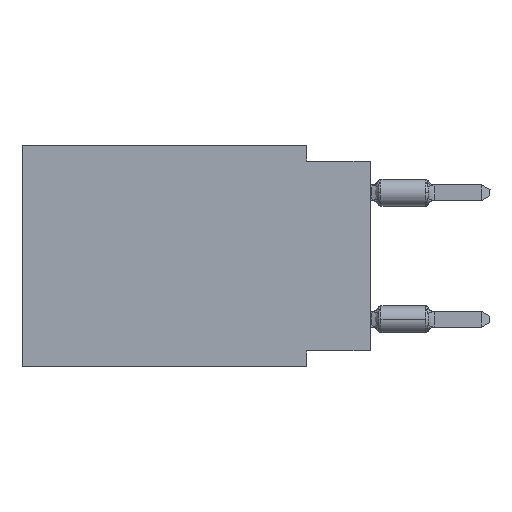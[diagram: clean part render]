
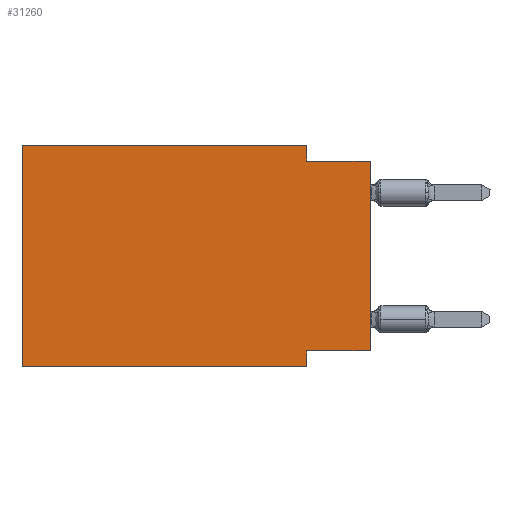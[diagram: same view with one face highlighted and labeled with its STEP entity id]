
A CAD part, left-side view. The second image highlights one B-rep face of the part: STEP entity #31260.
In plain terms, the highlighted planar face has unit normal (-1, 0, 0).
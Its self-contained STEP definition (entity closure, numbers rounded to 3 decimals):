
#143 = DIRECTION ( 'NONE',  ( 0., -1., 0. ) ) ;
#1596 = LINE ( 'NONE', #15163, #25583 ) ;
#1943 = EDGE_CURVE ( 'NONE', #33168, #24580, #10604, .T. ) ;
#2580 = FACE_OUTER_BOUND ( 'NONE', #4321, .T. ) ;
#3035 = VECTOR ( 'NONE', #9583, 1000. ) ;
#3718 = EDGE_CURVE ( 'NONE', #33021, #20253, #37984, .T. ) ;
#4321 = EDGE_LOOP ( 'NONE', ( #15997, #19466, #8358, #24351, #36821, #16368, #6652, #5869 ) ) ;
#4835 = DIRECTION ( 'NONE',  ( 0., 0., -1. ) ) ;
#5869 = ORIENTED_EDGE ( 'NONE', *, *, #16274, .F. ) ;
#6652 = ORIENTED_EDGE ( 'NONE', *, *, #42197, .F. ) ;
#6726 = CARTESIAN_POINT ( 'NONE',  ( 0., 2.54, -8.255 ) ) ;
#7044 = VECTOR ( 'NONE', #23242, 1000. ) ;
#8358 = ORIENTED_EDGE ( 'NONE', *, *, #13438, .F. ) ;
#8679 = VECTOR ( 'NONE', #29029, 1000. ) ;
#8822 = PLANE ( 'NONE',  #34450 ) ;
#9538 = CARTESIAN_POINT ( 'NONE',  ( 0., 2.54, -0.635 ) ) ;
#9583 = DIRECTION ( 'NONE',  ( 0., -1., 0. ) ) ;
#10604 = LINE ( 'NONE', #37695, #11522 ) ;
#11522 = VECTOR ( 'NONE', #143, 1000. ) ;
#11567 = LINE ( 'NONE', #34256, #15675 ) ;
#13027 = DIRECTION ( 'NONE',  ( 1., 0., 0. ) ) ;
#13438 = EDGE_CURVE ( 'NONE', #24580, #42688, #38391, .T. ) ;
#13461 = LINE ( 'NONE', #16352, #7044 ) ;
#14461 = DIRECTION ( 'NONE',  ( 0., 0., -1. ) ) ;
#15055 = CARTESIAN_POINT ( 'NONE',  ( 0., 2.54, 0. ) ) ;
#15163 = CARTESIAN_POINT ( 'NONE',  ( 0., 13.97, 0. ) ) ;
#15467 = CARTESIAN_POINT ( 'NONE',  ( 0., 0., 0. ) ) ;
#15601 = DIRECTION ( 'NONE',  ( 0., 1., 0. ) ) ;
#15675 = VECTOR ( 'NONE', #14461, 1000. ) ;
#15825 = CARTESIAN_POINT ( 'NONE',  ( 0., 0., -8.255 ) ) ;
#15997 = ORIENTED_EDGE ( 'NONE', *, *, #3718, .T. ) ;
#16274 = EDGE_CURVE ( 'NONE', #33021, #35080, #36049, .T. ) ;
#16352 = CARTESIAN_POINT ( 'NONE',  ( 0., 0., -0.635 ) ) ;
#16368 = ORIENTED_EDGE ( 'NONE', *, *, #20958, .T. ) ;
#18544 = CARTESIAN_POINT ( 'NONE',  ( 0., 13.97, -8.89 ) ) ;
#19466 = ORIENTED_EDGE ( 'NONE', *, *, #28152, .F. ) ;
#20253 = VERTEX_POINT ( 'NONE', #22331 ) ;
#20958 = EDGE_CURVE ( 'NONE', #43331, #32548, #36255, .T. ) ;
#22331 = CARTESIAN_POINT ( 'NONE',  ( 0., 0., -0.635 ) ) ;
#23242 = DIRECTION ( 'NONE',  ( 0., -1., 0. ) ) ;
#24351 = ORIENTED_EDGE ( 'NONE', *, *, #1943, .F. ) ;
#24580 = VERTEX_POINT ( 'NONE', #38920 ) ;
#24868 = VECTOR ( 'NONE', #4835, 1000. ) ;
#25583 = VECTOR ( 'NONE', #38922, 1000. ) ;
#26576 = DIRECTION ( 'NONE',  ( 0., 0., -1. ) ) ;
#26583 = CARTESIAN_POINT ( 'NONE',  ( 0., 2.54, -8.89 ) ) ;
#28152 = EDGE_CURVE ( 'NONE', #42688, #20253, #13461, .T. ) ;
#29029 = DIRECTION ( 'NONE',  ( 0., 0., 1. ) ) ;
#29907 = CARTESIAN_POINT ( 'NONE',  ( 0., 13.97, 0. ) ) ;
#31260 = ADVANCED_FACE ( 'NONE', ( #2580 ), #8822, .F. ) ;
#32548 = VERTEX_POINT ( 'NONE', #26583 ) ;
#33021 = VERTEX_POINT ( 'NONE', #40290 ) ;
#33168 = VERTEX_POINT ( 'NONE', #42041 ) ;
#34256 = CARTESIAN_POINT ( 'NONE',  ( 0., 2.54, -8.89 ) ) ;
#34450 = AXIS2_PLACEMENT_3D ( 'NONE', #29907, #13027, #26576 ) ;
#35080 = VERTEX_POINT ( 'NONE', #6726 ) ;
#36049 = LINE ( 'NONE', #15825, #37717 ) ;
#36255 = LINE ( 'NONE', #18544, #3035 ) ;
#36821 = ORIENTED_EDGE ( 'NONE', *, *, #40822, .F. ) ;
#37695 = CARTESIAN_POINT ( 'NONE',  ( 0., 13.97, 0. ) ) ;
#37717 = VECTOR ( 'NONE', #15601, 1000. ) ;
#37984 = LINE ( 'NONE', #15467, #8679 ) ;
#38391 = LINE ( 'NONE', #15055, #24868 ) ;
#38920 = CARTESIAN_POINT ( 'NONE',  ( 0., 2.54, 0. ) ) ;
#38922 = DIRECTION ( 'NONE',  ( 0., 0., 1. ) ) ;
#40290 = CARTESIAN_POINT ( 'NONE',  ( 0., 0., -8.255 ) ) ;
#40794 = CARTESIAN_POINT ( 'NONE',  ( 0., 13.97, -8.89 ) ) ;
#40822 = EDGE_CURVE ( 'NONE', #43331, #33168, #1596, .T. ) ;
#42041 = CARTESIAN_POINT ( 'NONE',  ( 0., 13.97, 0. ) ) ;
#42197 = EDGE_CURVE ( 'NONE', #35080, #32548, #11567, .T. ) ;
#42688 = VERTEX_POINT ( 'NONE', #9538 ) ;
#43331 = VERTEX_POINT ( 'NONE', #40794 ) ;
